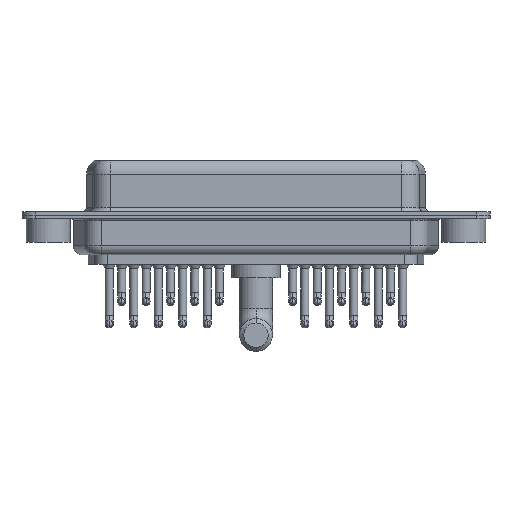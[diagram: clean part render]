
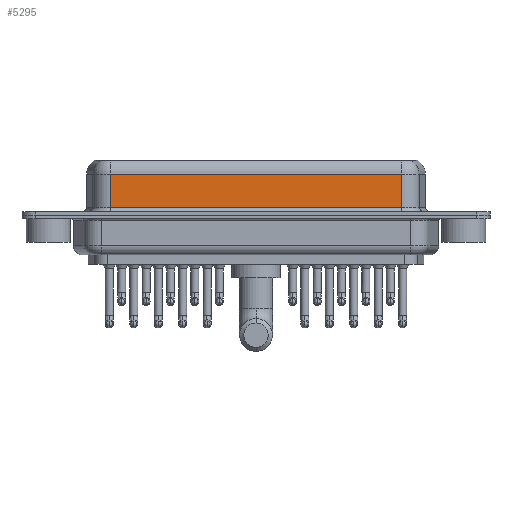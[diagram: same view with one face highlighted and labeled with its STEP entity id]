
A CAD part, front view. The second image highlights one B-rep face of the part: STEP entity #5295.
In plain terms, the highlighted planar face has unit normal (0, -1, 0).
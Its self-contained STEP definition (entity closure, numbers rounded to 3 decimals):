
#88 = CARTESIAN_POINT ( 'NONE',  ( 40.037, -3.95, 0.9 ) ) ;
#733 = VERTEX_POINT ( 'NONE', #9635 ) ;
#1170 = CARTESIAN_POINT ( 'NONE',  ( 7.013, -3.95, 6.4 ) ) ;
#1470 = PLANE ( 'NONE',  #18944 ) ;
#1800 = VERTEX_POINT ( 'NONE', #20476 ) ;
#1838 = VECTOR ( 'NONE', #19432, 1000. ) ;
#2387 = ORIENTED_EDGE ( 'NONE', *, *, #6709, .T. ) ;
#2545 = VERTEX_POINT ( 'NONE', #16639 ) ;
#3144 = DIRECTION ( 'NONE',  ( 0., 0., -1. ) ) ;
#3159 = ORIENTED_EDGE ( 'NONE', *, *, #22026, .T. ) ;
#3306 = CARTESIAN_POINT ( 'NONE',  ( 40.037, -3.95, 6.4 ) ) ;
#3376 = ORIENTED_EDGE ( 'NONE', *, *, #4111, .F. ) ;
#4111 = EDGE_CURVE ( 'NONE', #1800, #22265, #12134, .T. ) ;
#5295 = ADVANCED_FACE ( 'NONE', ( #11960 ), #1470, .F. ) ;
#6703 = LINE ( 'NONE', #1170, #19512 ) ;
#6709 = EDGE_CURVE ( 'NONE', #733, #22265, #12880, .T. ) ;
#8024 = LINE ( 'NONE', #19550, #1838 ) ;
#9635 = CARTESIAN_POINT ( 'NONE',  ( 7.013, -3.95, 0.9 ) ) ;
#9988 = DIRECTION ( 'NONE',  ( 0., 0., 1. ) ) ;
#11960 = FACE_OUTER_BOUND ( 'NONE', #12537, .T. ) ;
#12134 = LINE ( 'NONE', #18901, #22537 ) ;
#12537 = EDGE_LOOP ( 'NONE', ( #3376, #3159, #13005, #2387 ) ) ;
#12880 = LINE ( 'NONE', #16449, #22578 ) ;
#13005 = ORIENTED_EDGE ( 'NONE', *, *, #14959, .T. ) ;
#13717 = DIRECTION ( 'NONE',  ( 0., 0., -1. ) ) ;
#14959 = EDGE_CURVE ( 'NONE', #2545, #733, #6703, .T. ) ;
#16449 = CARTESIAN_POINT ( 'NONE',  ( 40.037, -3.95, 0.9 ) ) ;
#16639 = CARTESIAN_POINT ( 'NONE',  ( 7.013, -3.95, 4.65 ) ) ;
#17835 = DIRECTION ( 'NONE',  ( 1., 0., 0. ) ) ;
#18901 = CARTESIAN_POINT ( 'NONE',  ( 40.037, -3.95, 6.4 ) ) ;
#18944 = AXIS2_PLACEMENT_3D ( 'NONE', #3306, #22257, #9988 ) ;
#19432 = DIRECTION ( 'NONE',  ( -1., 0., 0. ) ) ;
#19512 = VECTOR ( 'NONE', #13717, 1000. ) ;
#19550 = CARTESIAN_POINT ( 'NONE',  ( 40.037, -3.95, 4.65 ) ) ;
#20476 = CARTESIAN_POINT ( 'NONE',  ( 40.037, -3.95, 4.65 ) ) ;
#22026 = EDGE_CURVE ( 'NONE', #1800, #2545, #8024, .T. ) ;
#22257 = DIRECTION ( 'NONE',  ( 0., 1., 0. ) ) ;
#22265 = VERTEX_POINT ( 'NONE', #88 ) ;
#22537 = VECTOR ( 'NONE', #3144, 1000. ) ;
#22578 = VECTOR ( 'NONE', #17835, 1000. ) ;
